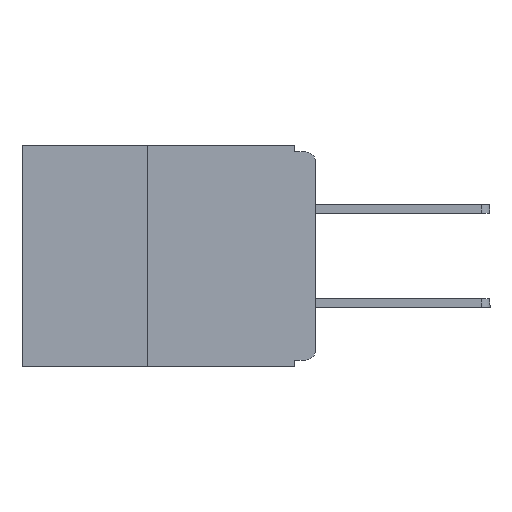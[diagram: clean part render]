
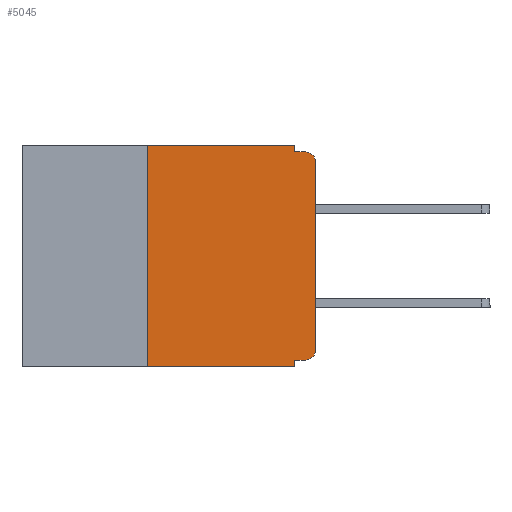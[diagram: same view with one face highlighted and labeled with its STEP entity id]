
A CAD part, left-side view. The second image highlights one B-rep face of the part: STEP entity #5045.
In plain terms, the highlighted planar face has unit normal (-1, 0, 0).
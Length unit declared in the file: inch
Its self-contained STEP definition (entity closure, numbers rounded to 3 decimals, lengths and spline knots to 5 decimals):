
#18 = ORIENTED_EDGE ( 'NONE', *, *, #4793, .F. ) ;
#235 = LINE ( 'NONE', #8747, #5338 ) ;
#455 = VECTOR ( 'NONE', #9217, 39.37008 ) ;
#578 = CARTESIAN_POINT ( 'NONE',  ( 0., 0., 0. ) ) ;
#615 = DIRECTION ( 'NONE',  ( 0., 0., 1. ) ) ;
#1037 = VECTOR ( 'NONE', #3405, 39.37008 ) ;
#1388 = EDGE_LOOP ( 'NONE', ( #2176, #5148, #18, #6067, #11308, #11571, #2025, #9637, #9893, #2664 ) ) ;
#1624 = VECTOR ( 'NONE', #2993, 39.37008 ) ;
#2025 = ORIENTED_EDGE ( 'NONE', *, *, #7090, .T. ) ;
#2176 = ORIENTED_EDGE ( 'NONE', *, *, #4375, .T. ) ;
#2216 = VERTEX_POINT ( 'NONE', #9355 ) ;
#2452 = CIRCLE ( 'NONE', #6153, 0.015 ) ;
#2533 = CARTESIAN_POINT ( 'NONE',  ( 0., 0.031, -0.33 ) ) ;
#2664 = ORIENTED_EDGE ( 'NONE', *, *, #5869, .T. ) ;
#2737 = VERTEX_POINT ( 'NONE', #3148 ) ;
#2957 = EDGE_CURVE ( 'NONE', #10783, #7856, #235, .T. ) ;
#2993 = DIRECTION ( 'NONE',  ( 0., -1., 0. ) ) ;
#3099 = VERTEX_POINT ( 'NONE', #5221 ) ;
#3148 = CARTESIAN_POINT ( 'NONE',  ( 0., 0.031, -0.33 ) ) ;
#3220 = LINE ( 'NONE', #2533, #455 ) ;
#3256 = CARTESIAN_POINT ( 'NONE',  ( 0., 0.015, -0.305 ) ) ;
#3405 = DIRECTION ( 'NONE',  ( 0., -1., 0. ) ) ;
#3423 = VECTOR ( 'NONE', #5165, 39.37008 ) ;
#3710 = LINE ( 'NONE', #4162, #3423 ) ;
#3713 = CARTESIAN_POINT ( 'NONE',  ( 0., 0.015, -0.025 ) ) ;
#3945 = VERTEX_POINT ( 'NONE', #5033 ) ;
#4000 = CARTESIAN_POINT ( 'NONE',  ( 0., 0.031, 0. ) ) ;
#4116 = VERTEX_POINT ( 'NONE', #11505 ) ;
#4162 = CARTESIAN_POINT ( 'NONE',  ( 0., 0., -0.32 ) ) ;
#4193 = FACE_OUTER_BOUND ( 'NONE', #1388, .T. ) ;
#4238 = DIRECTION ( 'NONE',  ( 0., 0., -1. ) ) ;
#4375 = EDGE_CURVE ( 'NONE', #2216, #3099, #9348, .T. ) ;
#4608 = VECTOR ( 'NONE', #8700, 39.37008 ) ;
#4726 = DIRECTION ( 'NONE',  ( 0., 0., -1. ) ) ;
#4793 = EDGE_CURVE ( 'NONE', #3945, #4116, #6365, .T. ) ;
#5033 = CARTESIAN_POINT ( 'NONE',  ( 0., 0.031, -0.01 ) ) ;
#5045 = ADVANCED_FACE ( 'NONE', ( #4193 ), #5686, .F. ) ;
#5055 = CARTESIAN_POINT ( 'NONE',  ( 0., 0.25, -0.33 ) ) ;
#5148 = ORIENTED_EDGE ( 'NONE', *, *, #5523, .T. ) ;
#5152 = VERTEX_POINT ( 'NONE', #12034 ) ;
#5165 = DIRECTION ( 'NONE',  ( 0., 1., 0. ) ) ;
#5221 = CARTESIAN_POINT ( 'NONE',  ( 0., 0., -0.025 ) ) ;
#5306 = EDGE_CURVE ( 'NONE', #5152, #8643, #3710, .T. ) ;
#5338 = VECTOR ( 'NONE', #6460, 39.37008 ) ;
#5344 = CARTESIAN_POINT ( 'NONE',  ( 0., 0., -0.01 ) ) ;
#5382 = LINE ( 'NONE', #11628, #8206 ) ;
#5523 = EDGE_CURVE ( 'NONE', #3099, #4116, #6491, .T. ) ;
#5686 = PLANE ( 'NONE',  #9853 ) ;
#5869 = EDGE_CURVE ( 'NONE', #5152, #2216, #2452, .T. ) ;
#6067 = ORIENTED_EDGE ( 'NONE', *, *, #6769, .F. ) ;
#6153 = AXIS2_PLACEMENT_3D ( 'NONE', #3256, #9813, #4238 ) ;
#6365 = LINE ( 'NONE', #5344, #1037 ) ;
#6460 = DIRECTION ( 'NONE',  ( 0., -1., 0. ) ) ;
#6491 = CIRCLE ( 'NONE', #7664, 0.015 ) ;
#6707 = DIRECTION ( 'NONE',  ( 0., 0., -1. ) ) ;
#6769 = EDGE_CURVE ( 'NONE', #7856, #3945, #5382, .T. ) ;
#7069 = EDGE_CURVE ( 'NONE', #7886, #10783, #7493, .T. ) ;
#7090 = EDGE_CURVE ( 'NONE', #7886, #2737, #9294, .T. ) ;
#7466 = EDGE_CURVE ( 'NONE', #8643, #2737, #3220, .T. ) ;
#7493 = LINE ( 'NONE', #7755, #4608 ) ;
#7664 = AXIS2_PLACEMENT_3D ( 'NONE', #3713, #10206, #4726 ) ;
#7755 = CARTESIAN_POINT ( 'NONE',  ( 0., 0.25, -0.33 ) ) ;
#7830 = CARTESIAN_POINT ( 'NONE',  ( 0., 0.437, -0.33 ) ) ;
#7856 = VERTEX_POINT ( 'NONE', #4000 ) ;
#7886 = VERTEX_POINT ( 'NONE', #5055 ) ;
#8206 = VECTOR ( 'NONE', #10805, 39.37008 ) ;
#8643 = VERTEX_POINT ( 'NONE', #9009 ) ;
#8700 = DIRECTION ( 'NONE',  ( 0., 0., 1. ) ) ;
#8747 = CARTESIAN_POINT ( 'NONE',  ( 0., 0.437, 0. ) ) ;
#9009 = CARTESIAN_POINT ( 'NONE',  ( 0., 0.031, -0.32 ) ) ;
#9217 = DIRECTION ( 'NONE',  ( 0., 0., -1. ) ) ;
#9294 = LINE ( 'NONE', #7830, #1624 ) ;
#9348 = LINE ( 'NONE', #578, #11047 ) ;
#9355 = CARTESIAN_POINT ( 'NONE',  ( 0., 0., -0.305 ) ) ;
#9637 = ORIENTED_EDGE ( 'NONE', *, *, #7466, .F. ) ;
#9813 = DIRECTION ( 'NONE',  ( -1., 0., 0. ) ) ;
#9853 = AXIS2_PLACEMENT_3D ( 'NONE', #11056, #11895, #6707 ) ;
#9893 = ORIENTED_EDGE ( 'NONE', *, *, #5306, .F. ) ;
#10047 = CARTESIAN_POINT ( 'NONE',  ( 0., 0.25, 0. ) ) ;
#10206 = DIRECTION ( 'NONE',  ( -1., 0., 0. ) ) ;
#10783 = VERTEX_POINT ( 'NONE', #10047 ) ;
#10805 = DIRECTION ( 'NONE',  ( 0., 0., -1. ) ) ;
#11047 = VECTOR ( 'NONE', #615, 39.37008 ) ;
#11056 = CARTESIAN_POINT ( 'NONE',  ( 0., 0.437, 0. ) ) ;
#11308 = ORIENTED_EDGE ( 'NONE', *, *, #2957, .F. ) ;
#11505 = CARTESIAN_POINT ( 'NONE',  ( 0., 0.015, -0.01 ) ) ;
#11571 = ORIENTED_EDGE ( 'NONE', *, *, #7069, .F. ) ;
#11628 = CARTESIAN_POINT ( 'NONE',  ( 0., 0.031, 0. ) ) ;
#11895 = DIRECTION ( 'NONE',  ( 1., 0., 0. ) ) ;
#12034 = CARTESIAN_POINT ( 'NONE',  ( 0., 0.015, -0.32 ) ) ;
